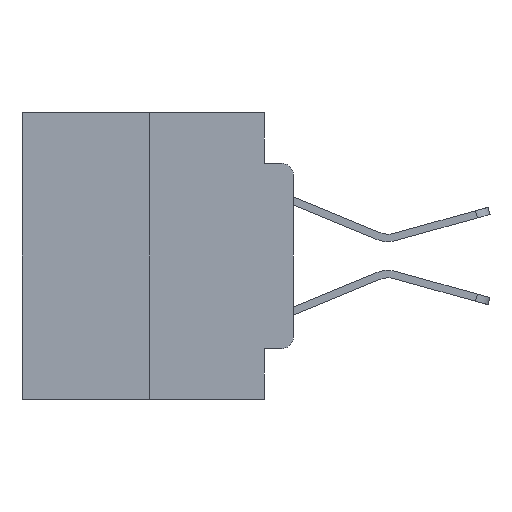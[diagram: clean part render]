
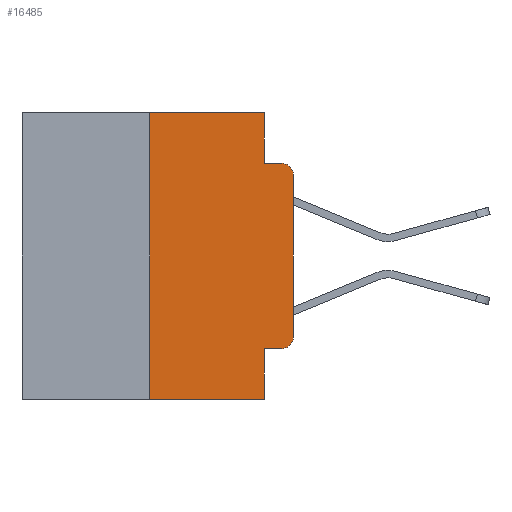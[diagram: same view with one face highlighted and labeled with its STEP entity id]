
A CAD part, left-side view. The second image highlights one B-rep face of the part: STEP entity #16485.
In plain terms, the highlighted planar face has unit normal (-1, 0, 0).
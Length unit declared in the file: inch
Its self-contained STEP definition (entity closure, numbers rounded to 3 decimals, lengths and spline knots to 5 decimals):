
#256 = ORIENTED_EDGE ( 'NONE', *, *, #23753, .F. ) ;
#760 = CARTESIAN_POINT ( 'NONE',  ( 0., 0.02, -0.3915 ) ) ;
#777 = CARTESIAN_POINT ( 'NONE',  ( 0., 0.02, -0.1085 ) ) ;
#1026 = AXIS2_PLACEMENT_3D ( 'NONE', #10190, #12341, #25164 ) ;
#1807 = EDGE_CURVE ( 'NONE', #7669, #4003, #17986, .T. ) ;
#1916 = ORIENTED_EDGE ( 'NONE', *, *, #9882, .T. ) ;
#2033 = DIRECTION ( 'NONE',  ( 0., -1., 0. ) ) ;
#2297 = CARTESIAN_POINT ( 'NONE',  ( 0., 0.473, -0.5 ) ) ;
#2931 = DIRECTION ( 'NONE',  ( -1., 0., 0. ) ) ;
#3012 = ORIENTED_EDGE ( 'NONE', *, *, #15189, .T. ) ;
#3220 = ORIENTED_EDGE ( 'NONE', *, *, #13776, .T. ) ;
#3726 = ORIENTED_EDGE ( 'NONE', *, *, #15755, .F. ) ;
#4003 = VERTEX_POINT ( 'NONE', #14901 ) ;
#4196 = FACE_OUTER_BOUND ( 'NONE', #5557, .T. ) ;
#4356 = VERTEX_POINT ( 'NONE', #13884 ) ;
#4563 = ORIENTED_EDGE ( 'NONE', *, *, #1807, .T. ) ;
#5505 = VERTEX_POINT ( 'NONE', #9349 ) ;
#5557 = EDGE_LOOP ( 'NONE', ( #13054, #4563, #8540, #256, #27279, #3726, #1916, #23779, #3012, #3220 ) ) ;
#5663 = CARTESIAN_POINT ( 'NONE',  ( 0., 0.473, 0. ) ) ;
#5853 = LINE ( 'NONE', #17795, #7216 ) ;
#6882 = CARTESIAN_POINT ( 'NONE',  ( 0., 0.02, -0.4115 ) ) ;
#6916 = EDGE_CURVE ( 'NONE', #4356, #4003, #17722, .T. ) ;
#7216 = VECTOR ( 'NONE', #21741, 39.37008 ) ;
#7634 = DIRECTION ( 'NONE',  ( 0., -1., 0. ) ) ;
#7669 = VERTEX_POINT ( 'NONE', #26110 ) ;
#7684 = CARTESIAN_POINT ( 'NONE',  ( 0., 0.051, -0.4115 ) ) ;
#8033 = PLANE ( 'NONE',  #1026 ) ;
#8540 = ORIENTED_EDGE ( 'NONE', *, *, #6916, .F. ) ;
#8659 = DIRECTION ( 'NONE',  ( 0., -1., 0. ) ) ;
#9148 = DIRECTION ( 'NONE',  ( 0., 0., -1. ) ) ;
#9349 = CARTESIAN_POINT ( 'NONE',  ( 0., 0.051, 0. ) ) ;
#9363 = VECTOR ( 'NONE', #17371, 39.37008 ) ;
#9614 = VECTOR ( 'NONE', #8659, 39.37008 ) ;
#9882 = EDGE_CURVE ( 'NONE', #19555, #26622, #18691, .T. ) ;
#10190 = CARTESIAN_POINT ( 'NONE',  ( 0., 0.473, 0. ) ) ;
#10244 = LINE ( 'NONE', #24401, #26132 ) ;
#10318 = DIRECTION ( 'NONE',  ( 0., 0., 1. ) ) ;
#10322 = VERTEX_POINT ( 'NONE', #7684 ) ;
#10871 = CIRCLE ( 'NONE', #14722, 0.02 ) ;
#11169 = CARTESIAN_POINT ( 'NONE',  ( 0., 0.25, 0. ) ) ;
#11433 = VERTEX_POINT ( 'NONE', #20377 ) ;
#12341 = DIRECTION ( 'NONE',  ( 1., 0., 0. ) ) ;
#13054 = ORIENTED_EDGE ( 'NONE', *, *, #13675, .T. ) ;
#13675 = EDGE_CURVE ( 'NONE', #11433, #7669, #5853, .T. ) ;
#13776 = EDGE_CURVE ( 'NONE', #17305, #11433, #10871, .T. ) ;
#13884 = CARTESIAN_POINT ( 'NONE',  ( 0., 0.051, -0.0885 ) ) ;
#13902 = VECTOR ( 'NONE', #10318, 39.37008 ) ;
#14722 = AXIS2_PLACEMENT_3D ( 'NONE', #760, #21836, #9148 ) ;
#14901 = CARTESIAN_POINT ( 'NONE',  ( 0., 0.02, -0.0885 ) ) ;
#15189 = EDGE_CURVE ( 'NONE', #10322, #17305, #18241, .T. ) ;
#15755 = EDGE_CURVE ( 'NONE', #19555, #22300, #19506, .T. ) ;
#16327 = DIRECTION ( 'NONE',  ( 0., 0., -1. ) ) ;
#16485 = ADVANCED_FACE ( 'NONE', ( #4196 ), #8033, .F. ) ;
#17062 = VECTOR ( 'NONE', #23718, 39.37008 ) ;
#17305 = VERTEX_POINT ( 'NONE', #6882 ) ;
#17371 = DIRECTION ( 'NONE',  ( 0., 0., -1. ) ) ;
#17722 = LINE ( 'NONE', #21601, #17062 ) ;
#17795 = CARTESIAN_POINT ( 'NONE',  ( 0., 0., 0. ) ) ;
#17986 = CIRCLE ( 'NONE', #26837, 0.02 ) ;
#18241 = LINE ( 'NONE', #21335, #9614 ) ;
#18691 = LINE ( 'NONE', #2297, #26275 ) ;
#18993 = LINE ( 'NONE', #5663, #26911 ) ;
#19121 = CARTESIAN_POINT ( 'NONE',  ( 0., 0.25, -0.5 ) ) ;
#19251 = CARTESIAN_POINT ( 'NONE',  ( 0., 0.051, -0.5 ) ) ;
#19506 = LINE ( 'NONE', #22988, #13902 ) ;
#19555 = VERTEX_POINT ( 'NONE', #19121 ) ;
#20096 = DIRECTION ( 'NONE',  ( 0., 0., -1. ) ) ;
#20377 = CARTESIAN_POINT ( 'NONE',  ( 0., 0., -0.3915 ) ) ;
#21335 = CARTESIAN_POINT ( 'NONE',  ( 0., 0.051, -0.4115 ) ) ;
#21601 = CARTESIAN_POINT ( 'NONE',  ( 0., 0.051, -0.0885 ) ) ;
#21741 = DIRECTION ( 'NONE',  ( 0., 0., 1. ) ) ;
#21836 = DIRECTION ( 'NONE',  ( -1., 0., 0. ) ) ;
#22300 = VERTEX_POINT ( 'NONE', #11169 ) ;
#22988 = CARTESIAN_POINT ( 'NONE',  ( 0., 0.25, 0. ) ) ;
#23327 = EDGE_CURVE ( 'NONE', #22300, #5505, #18993, .T. ) ;
#23581 = LINE ( 'NONE', #23720, #9363 ) ;
#23718 = DIRECTION ( 'NONE',  ( 0., -1., 0. ) ) ;
#23720 = CARTESIAN_POINT ( 'NONE',  ( 0., 0.051, 0. ) ) ;
#23753 = EDGE_CURVE ( 'NONE', #5505, #4356, #23581, .T. ) ;
#23779 = ORIENTED_EDGE ( 'NONE', *, *, #25875, .F. ) ;
#24401 = CARTESIAN_POINT ( 'NONE',  ( 0., 0.051, 0. ) ) ;
#25164 = DIRECTION ( 'NONE',  ( 0., 0., -1. ) ) ;
#25875 = EDGE_CURVE ( 'NONE', #10322, #26622, #10244, .T. ) ;
#26110 = CARTESIAN_POINT ( 'NONE',  ( 0., 0., -0.1085 ) ) ;
#26132 = VECTOR ( 'NONE', #16327, 39.37008 ) ;
#26275 = VECTOR ( 'NONE', #2033, 39.37008 ) ;
#26622 = VERTEX_POINT ( 'NONE', #19251 ) ;
#26837 = AXIS2_PLACEMENT_3D ( 'NONE', #777, #2931, #20096 ) ;
#26911 = VECTOR ( 'NONE', #7634, 39.37008 ) ;
#27279 = ORIENTED_EDGE ( 'NONE', *, *, #23327, .F. ) ;
